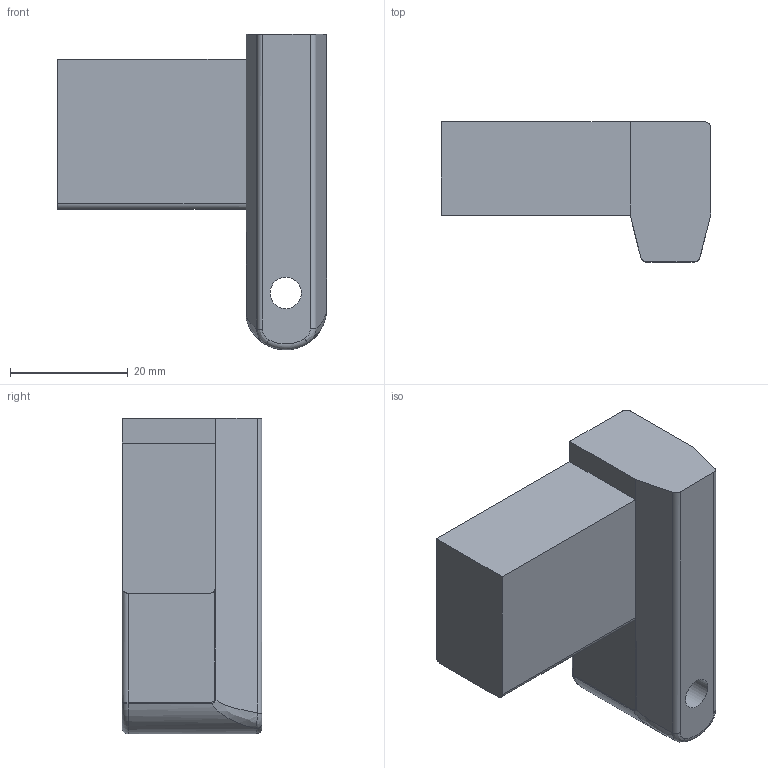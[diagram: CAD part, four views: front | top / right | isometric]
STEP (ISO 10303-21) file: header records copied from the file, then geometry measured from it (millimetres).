
FILE_DESCRIPTION (( 'STEP AP203' ), '1' );
FILE_NAME ('MOD9_G36_stock_lock.STEP', '2020-07-07T01:49:00', ( '' ), ( '' ), 'SwSTEP 2.0', 'SolidWorks 2016', '' );
FILE_SCHEMA (( 'CONFIG_CONTROL_DESIGN' ));
Length unit declared in the file: millimetre
Products named in the file (1): MOD9_G36_stock_lock
Bounding box: 45.75 x 23.76 x 53.67 mm (x, y, z)
Volume: 28584.7 mm3; surface area: 7205.2 mm2
Topology: 1 solids, 1 shells, 35 faces, 86 edges, 52 vertices
Faces by surface type: plane 15, cylinder 11, bspline 5, torus 2, sphere 1, cone 1
Full cylindrical faces by diameter (mm): 5.346 x1
Entity records: 1218 total; most frequent: CARTESIAN_POINT 361, ORIENTED_EDGE 166, DIRECTION 150, EDGE_CURVE 83, AXIS2_PLACEMENT_3D 53, VERTEX_POINT 52, VECTOR 44, LINE 44
